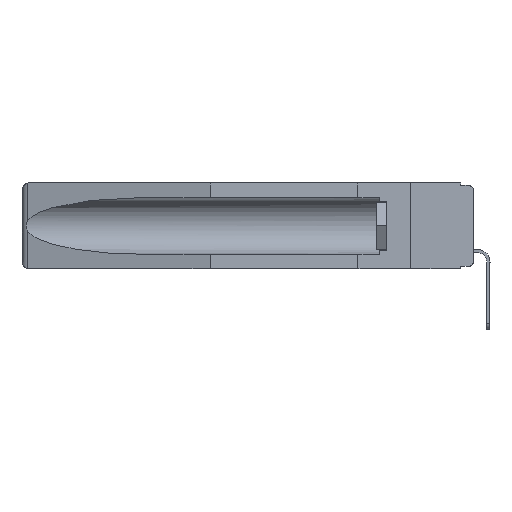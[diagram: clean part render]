
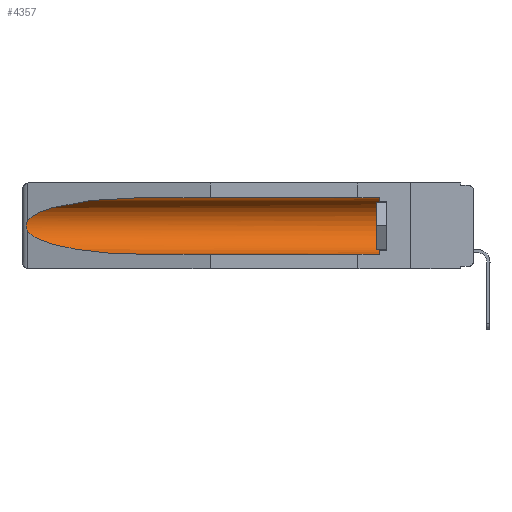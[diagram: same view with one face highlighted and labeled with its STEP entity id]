
A CAD part, left-side view. The second image highlights one B-rep face of the part: STEP entity #4357.
In plain terms, the highlighted cylindrical face has radius 2.857 mm (diameter 5.715 mm), a partial arc.
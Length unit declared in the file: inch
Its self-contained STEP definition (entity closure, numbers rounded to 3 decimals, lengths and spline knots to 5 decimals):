
#216 = CARTESIAN_POINT ( 'NONE',  ( 0.21114, 1.30732, -0.284 ) ) ;
#473 = CARTESIAN_POINT ( 'NONE',  ( 0.155, 1.07973, -0.284 ) ) ;
#939 = ORIENTED_EDGE ( 'NONE', *, *, #3121, .F. ) ;
#1163 =( BOUNDED_CURVE ( )  B_SPLINE_CURVE ( 3, ( #2525, #15876, #216, #473 ),
 .UNSPECIFIED., .F., .T. ) 
 B_SPLINE_CURVE_WITH_KNOTS ( ( 4, 4 ),
 ( 0.1948, 1.5708 ),
 .UNSPECIFIED. ) 
 CURVE ( )  GEOMETRIC_REPRESENTATION_ITEM ( )  RATIONAL_B_SPLINE_CURVE ( ( 1., 0.848, 0.848, 1. ) ) 
 REPRESENTATION_ITEM ( '' )  );
#1181 = B_SPLINE_CURVE_WITH_KNOTS ( 'NONE', 3,
 ( #17327, #7417, #16932, #25136, #15731, #1271, #14997, #11149, #1391, #9223 ),
 .UNSPECIFIED., .F., .F.,
 ( 4, 2, 2, 2, 4 ),
 ( 0., 0.00029, 0.00058, 0.00087, 0.00117 ),
 .UNSPECIFIED. ) ;
#1271 = CARTESIAN_POINT ( 'NONE',  ( 0.2675, 1.53308, -0.17534 ) ) ;
#1391 = CARTESIAN_POINT ( 'NONE',  ( 0.26597, 1.5296, -0.19026 ) ) ;
#2003 =( BOUNDED_CURVE ( )  B_SPLINE_CURVE ( 3, ( #2700, #15917, #16189, #13990 ),
 .UNSPECIFIED., .F., .T. ) 
 B_SPLINE_CURVE_WITH_KNOTS ( ( 4, 4 ),
 ( 4.71239, 6.08839 ),
 .UNSPECIFIED. ) 
 CURVE ( )  GEOMETRIC_REPRESENTATION_ITEM ( )  RATIONAL_B_SPLINE_CURVE ( ( 1., 0.848, 0.848, 1. ) ) 
 REPRESENTATION_ITEM ( '' )  );
#2470 = CARTESIAN_POINT ( 'NONE',  ( 0.26537, 1.52718, -0.19328 ) ) ;
#2525 = CARTESIAN_POINT ( 'NONE',  ( 0.26537, 1.52718, -0.19328 ) ) ;
#2700 = CARTESIAN_POINT ( 'NONE',  ( 0.155, 1.07973, -0.059 ) ) ;
#3121 = EDGE_CURVE ( 'NONE', #23727, #5610, #22013, .T. ) ;
#3230 = AXIS2_PLACEMENT_3D ( 'NONE', #20013, #18088, #23612 ) ;
#3588 = ORIENTED_EDGE ( 'NONE', *, *, #6107, .T. ) ;
#4079 = EDGE_CURVE ( 'NONE', #23727, #11369, #19712, .T. ) ;
#4357 = ADVANCED_FACE ( 'NONE', ( #5858 ), #7916, .F. ) ;
#4634 = EDGE_LOOP ( 'NONE', ( #13366, #24654, #3588, #939, #4813, #24809 ) ) ;
#4813 = ORIENTED_EDGE ( 'NONE', *, *, #4079, .T. ) ;
#4853 = DIRECTION ( 'NONE',  ( 0., -1., 0. ) ) ;
#5305 = CARTESIAN_POINT ( 'NONE',  ( 0.155, 0.126, -0.284 ) ) ;
#5610 = VERTEX_POINT ( 'NONE', #25148 ) ;
#5855 = VECTOR ( 'NONE', #7491, 39.37008 ) ;
#5858 = FACE_OUTER_BOUND ( 'NONE', #4634, .T. ) ;
#6107 = EDGE_CURVE ( 'NONE', #21321, #5610, #1163, .T. ) ;
#7381 = EDGE_CURVE ( 'NONE', #11369, #9940, #15595, .T. ) ;
#7417 = CARTESIAN_POINT ( 'NONE',  ( 0.26597, 1.52961, -0.15275 ) ) ;
#7491 = DIRECTION ( 'NONE',  ( 0., 1., 0. ) ) ;
#7916 = CYLINDRICAL_SURFACE ( 'NONE', #3230, 0.1125 ) ;
#8712 = CARTESIAN_POINT ( 'NONE',  ( 0.155, 0.126, -0.1715 ) ) ;
#9223 = CARTESIAN_POINT ( 'NONE',  ( 0.26537, 1.52718, -0.19328 ) ) ;
#9940 = VERTEX_POINT ( 'NONE', #24496 ) ;
#11149 = CARTESIAN_POINT ( 'NONE',  ( 0.26655, 1.53094, -0.18657 ) ) ;
#11369 = VERTEX_POINT ( 'NONE', #20216 ) ;
#12259 = DIRECTION ( 'NONE',  ( 0., 1., 0. ) ) ;
#13366 = ORIENTED_EDGE ( 'NONE', *, *, #17417, .T. ) ;
#13552 = AXIS2_PLACEMENT_3D ( 'NONE', #8712, #4853, #14626 ) ;
#13915 = EDGE_CURVE ( 'NONE', #17416, #21321, #1181, .T. ) ;
#13990 = CARTESIAN_POINT ( 'NONE',  ( 0.26537, 1.52718, -0.14972 ) ) ;
#14626 = DIRECTION ( 'NONE',  ( 0., 0., 1. ) ) ;
#14997 = CARTESIAN_POINT ( 'NONE',  ( 0.2673, 1.53269, -0.17917 ) ) ;
#15595 = LINE ( 'NONE', #21361, #5855 ) ;
#15731 = CARTESIAN_POINT ( 'NONE',  ( 0.2675, 1.53308, -0.16763 ) ) ;
#15876 = CARTESIAN_POINT ( 'NONE',  ( 0.25451, 1.48313, -0.24835 ) ) ;
#15917 = CARTESIAN_POINT ( 'NONE',  ( 0.21114, 1.30732, -0.059 ) ) ;
#16189 = CARTESIAN_POINT ( 'NONE',  ( 0.25451, 1.48313, -0.09465 ) ) ;
#16932 = CARTESIAN_POINT ( 'NONE',  ( 0.26654, 1.53092, -0.15636 ) ) ;
#17327 = CARTESIAN_POINT ( 'NONE',  ( 0.26537, 1.52718, -0.14972 ) ) ;
#17416 = VERTEX_POINT ( 'NONE', #18247 ) ;
#17417 = EDGE_CURVE ( 'NONE', #9940, #17416, #2003, .T. ) ;
#17925 = CARTESIAN_POINT ( 'NONE',  ( 0.155, -0.30754, -0.284 ) ) ;
#18088 = DIRECTION ( 'NONE',  ( 0., 1., 0. ) ) ;
#18247 = CARTESIAN_POINT ( 'NONE',  ( 0.26537, 1.52718, -0.14972 ) ) ;
#19461 = VECTOR ( 'NONE', #12259, 39.37008 ) ;
#19712 = CIRCLE ( 'NONE', #13552, 0.1125 ) ;
#20013 = CARTESIAN_POINT ( 'NONE',  ( 0.155, -0.30754, -0.1715 ) ) ;
#20216 = CARTESIAN_POINT ( 'NONE',  ( 0.155, 0.126, -0.059 ) ) ;
#21321 = VERTEX_POINT ( 'NONE', #2470 ) ;
#21361 = CARTESIAN_POINT ( 'NONE',  ( 0.155, -0.30754, -0.059 ) ) ;
#22013 = LINE ( 'NONE', #17925, #19461 ) ;
#23612 = DIRECTION ( 'NONE',  ( 0., 0., 1. ) ) ;
#23727 = VERTEX_POINT ( 'NONE', #5305 ) ;
#24496 = CARTESIAN_POINT ( 'NONE',  ( 0.155, 1.07973, -0.059 ) ) ;
#24654 = ORIENTED_EDGE ( 'NONE', *, *, #13915, .T. ) ;
#24809 = ORIENTED_EDGE ( 'NONE', *, *, #7381, .T. ) ;
#25136 = CARTESIAN_POINT ( 'NONE',  ( 0.2673, 1.5327, -0.16383 ) ) ;
#25148 = CARTESIAN_POINT ( 'NONE',  ( 0.155, 1.07973, -0.284 ) ) ;
